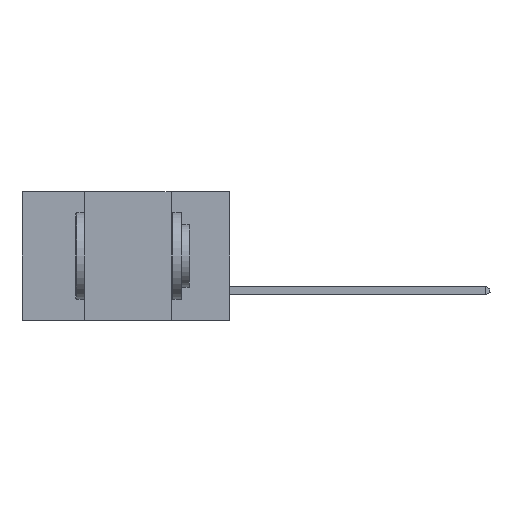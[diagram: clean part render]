
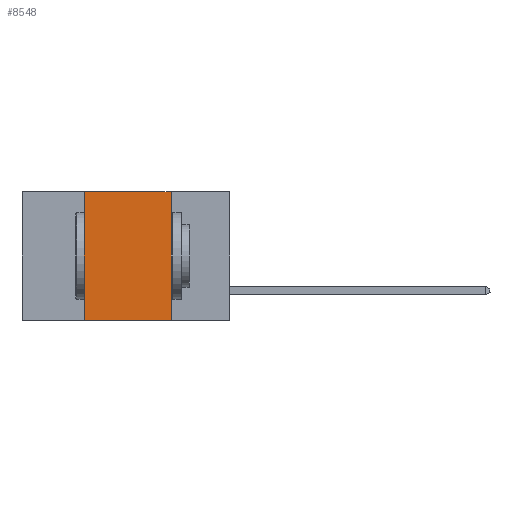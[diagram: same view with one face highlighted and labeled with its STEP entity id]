
A CAD part, left-side view. The second image highlights one B-rep face of the part: STEP entity #8548.
In plain terms, the highlighted planar face has unit normal (-1, 0, 0).
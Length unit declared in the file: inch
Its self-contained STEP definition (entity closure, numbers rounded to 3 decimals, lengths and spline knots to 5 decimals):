
#151 = VECTOR ( 'NONE', #17535, 39.37008 ) ;
#247 = CARTESIAN_POINT ( 'NONE',  ( 0., 0.6, -0.37 ) ) ;
#429 = EDGE_LOOP ( 'NONE', ( #23741, #4664, #19230, #12798 ) ) ;
#767 = CARTESIAN_POINT ( 'NONE',  ( 0., 0.17, 0. ) ) ;
#3060 = LINE ( 'NONE', #19274, #9958 ) ;
#3193 = VERTEX_POINT ( 'NONE', #20540 ) ;
#3758 = CARTESIAN_POINT ( 'NONE',  ( 0., 0.6, 0. ) ) ;
#4664 = ORIENTED_EDGE ( 'NONE', *, *, #18949, .F. ) ;
#7330 = DIRECTION ( 'NONE',  ( 1., 0., 0. ) ) ;
#8119 = VECTOR ( 'NONE', #12673, 39.37008 ) ;
#8548 = ADVANCED_FACE ( 'NONE', ( #22836 ), #19013, .F. ) ;
#8700 = CARTESIAN_POINT ( 'NONE',  ( 0., 0.42, 0. ) ) ;
#9864 = DIRECTION ( 'NONE',  ( 0., 0., 1. ) ) ;
#9958 = VECTOR ( 'NONE', #9864, 39.37008 ) ;
#10392 = VECTOR ( 'NONE', #19911, 39.37008 ) ;
#11222 = LINE ( 'NONE', #247, #151 ) ;
#12585 = CARTESIAN_POINT ( 'NONE',  ( 0., 0.6, 0. ) ) ;
#12592 = LINE ( 'NONE', #12585, #8119 ) ;
#12673 = DIRECTION ( 'NONE',  ( 0., -1., 0. ) ) ;
#12798 = ORIENTED_EDGE ( 'NONE', *, *, #22528, .T. ) ;
#14533 = EDGE_CURVE ( 'NONE', #3193, #20547, #24636, .T. ) ;
#15016 = CARTESIAN_POINT ( 'NONE',  ( 0., 0.42, -0.37 ) ) ;
#16801 = VERTEX_POINT ( 'NONE', #8700 ) ;
#17535 = DIRECTION ( 'NONE',  ( 0., -1., 0. ) ) ;
#18949 = EDGE_CURVE ( 'NONE', #16801, #3193, #12592, .T. ) ;
#19013 = PLANE ( 'NONE',  #20902 ) ;
#19230 = ORIENTED_EDGE ( 'NONE', *, *, #23175, .F. ) ;
#19274 = CARTESIAN_POINT ( 'NONE',  ( 0., 0.42, 0. ) ) ;
#19440 = CARTESIAN_POINT ( 'NONE',  ( 0., 0.17, -0.37 ) ) ;
#19911 = DIRECTION ( 'NONE',  ( 0., 0., -1. ) ) ;
#20540 = CARTESIAN_POINT ( 'NONE',  ( 0., 0.17, 0. ) ) ;
#20547 = VERTEX_POINT ( 'NONE', #19440 ) ;
#20902 = AXIS2_PLACEMENT_3D ( 'NONE', #3758, #7330, #22808 ) ;
#21184 = VERTEX_POINT ( 'NONE', #15016 ) ;
#22528 = EDGE_CURVE ( 'NONE', #21184, #20547, #11222, .T. ) ;
#22808 = DIRECTION ( 'NONE',  ( 0., 0., -1. ) ) ;
#22836 = FACE_OUTER_BOUND ( 'NONE', #429, .T. ) ;
#23175 = EDGE_CURVE ( 'NONE', #21184, #16801, #3060, .T. ) ;
#23741 = ORIENTED_EDGE ( 'NONE', *, *, #14533, .F. ) ;
#24636 = LINE ( 'NONE', #767, #10392 ) ;
